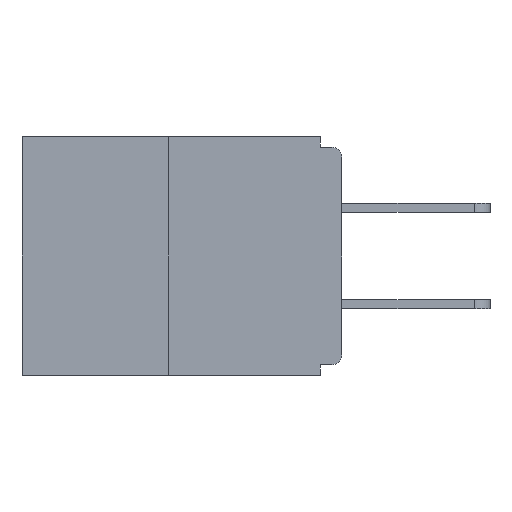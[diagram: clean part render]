
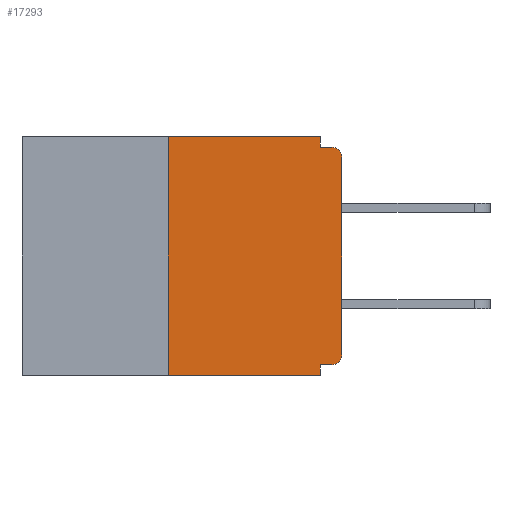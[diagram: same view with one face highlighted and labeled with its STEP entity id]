
A CAD part, left-side view. The second image highlights one B-rep face of the part: STEP entity #17293.
In plain terms, the highlighted planar face has unit normal (-1, 0, 0).
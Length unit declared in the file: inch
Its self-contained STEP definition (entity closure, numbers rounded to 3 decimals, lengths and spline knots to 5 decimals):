
#35 = CARTESIAN_POINT ( 'NONE',  ( 0., 0.25, 0. ) ) ;
#37 = ORIENTED_EDGE ( 'NONE', *, *, #15810, .F. ) ;
#222 = LINE ( 'NONE', #5067, #6453 ) ;
#289 = VECTOR ( 'NONE', #467, 39.37008 ) ;
#467 = DIRECTION ( 'NONE',  ( 0., 1., 0. ) ) ;
#476 = CARTESIAN_POINT ( 'NONE',  ( 0., 0.25, -0.343 ) ) ;
#492 = CARTESIAN_POINT ( 'NONE',  ( 0., 0., -0.015 ) ) ;
#697 = VECTOR ( 'NONE', #11536, 39.37008 ) ;
#717 = VERTEX_POINT ( 'NONE', #6315 ) ;
#784 = AXIS2_PLACEMENT_3D ( 'NONE', #18936, #14417, #8345 ) ;
#836 = LINE ( 'NONE', #3736, #14945 ) ;
#1163 = LINE ( 'NONE', #9948, #697 ) ;
#1172 = CARTESIAN_POINT ( 'NONE',  ( 0., 0., -0.313 ) ) ;
#1773 = EDGE_CURVE ( 'NONE', #6653, #7710, #836, .T. ) ;
#1789 = EDGE_CURVE ( 'NONE', #2468, #10516, #15435, .T. ) ;
#2468 = VERTEX_POINT ( 'NONE', #35 ) ;
#3152 = EDGE_LOOP ( 'NONE', ( #18760, #17387, #11220, #4796, #8653, #9577, #8104, #3454, #37, #15561 ) ) ;
#3274 = DIRECTION ( 'NONE',  ( -1., 0., 0. ) ) ;
#3454 = ORIENTED_EDGE ( 'NONE', *, *, #9477, .T. ) ;
#3498 = CARTESIAN_POINT ( 'NONE',  ( 0., 0., -0.328 ) ) ;
#3604 = DIRECTION ( 'NONE',  ( 0., -1., 0. ) ) ;
#3695 = CARTESIAN_POINT ( 'NONE',  ( 0., 0., 0. ) ) ;
#3736 = CARTESIAN_POINT ( 'NONE',  ( 0., 0.46, -0.343 ) ) ;
#3922 = CARTESIAN_POINT ( 'NONE',  ( 0., 0.46, 0. ) ) ;
#4766 = CARTESIAN_POINT ( 'NONE',  ( 0., 0.015, -0.03 ) ) ;
#4796 = ORIENTED_EDGE ( 'NONE', *, *, #15490, .F. ) ;
#5067 = CARTESIAN_POINT ( 'NONE',  ( 0., 0.031, 0. ) ) ;
#5096 = EDGE_CURVE ( 'NONE', #7377, #13472, #15283, .T. ) ;
#5201 = VECTOR ( 'NONE', #13180, 39.37008 ) ;
#5487 = EDGE_CURVE ( 'NONE', #10516, #18674, #222, .T. ) ;
#5579 = EDGE_CURVE ( 'NONE', #6653, #2468, #1163, .T. ) ;
#6140 = CARTESIAN_POINT ( 'NONE',  ( 0., 0., -0.03 ) ) ;
#6315 = CARTESIAN_POINT ( 'NONE',  ( 0., 0.015, -0.015 ) ) ;
#6453 = VECTOR ( 'NONE', #17282, 39.37008 ) ;
#6653 = VERTEX_POINT ( 'NONE', #476 ) ;
#6843 = AXIS2_PLACEMENT_3D ( 'NONE', #8447, #19269, #14647 ) ;
#7377 = VERTEX_POINT ( 'NONE', #18433 ) ;
#7611 = AXIS2_PLACEMENT_3D ( 'NONE', #4766, #3274, #15344 ) ;
#7710 = VERTEX_POINT ( 'NONE', #18407 ) ;
#8104 = ORIENTED_EDGE ( 'NONE', *, *, #18426, .T. ) ;
#8345 = DIRECTION ( 'NONE',  ( 0., 0., -1. ) ) ;
#8407 = DIRECTION ( 'NONE',  ( 0., 0., 1. ) ) ;
#8447 = CARTESIAN_POINT ( 'NONE',  ( 0., 0.46, 0. ) ) ;
#8653 = ORIENTED_EDGE ( 'NONE', *, *, #18342, .F. ) ;
#9157 = VECTOR ( 'NONE', #8407, 39.37008 ) ;
#9477 = EDGE_CURVE ( 'NONE', #18735, #717, #11991, .T. ) ;
#9518 = VECTOR ( 'NONE', #10223, 39.37008 ) ;
#9577 = ORIENTED_EDGE ( 'NONE', *, *, #5096, .T. ) ;
#9948 = CARTESIAN_POINT ( 'NONE',  ( 0., 0.25, 0. ) ) ;
#10217 = LINE ( 'NONE', #492, #19510 ) ;
#10223 = DIRECTION ( 'NONE',  ( 0., 0., -1. ) ) ;
#10516 = VERTEX_POINT ( 'NONE', #17755 ) ;
#11220 = ORIENTED_EDGE ( 'NONE', *, *, #1773, .T. ) ;
#11402 = DIRECTION ( 'NONE',  ( 0., -1., 0. ) ) ;
#11536 = DIRECTION ( 'NONE',  ( 0., 0., 1. ) ) ;
#11818 = VERTEX_POINT ( 'NONE', #12391 ) ;
#11991 = CIRCLE ( 'NONE', #7611, 0.015 ) ;
#12029 = LINE ( 'NONE', #3498, #289 ) ;
#12391 = CARTESIAN_POINT ( 'NONE',  ( 0., 0.031, -0.328 ) ) ;
#12835 = LINE ( 'NONE', #18020, #9518 ) ;
#13180 = DIRECTION ( 'NONE',  ( 0., -1., 0. ) ) ;
#13472 = VERTEX_POINT ( 'NONE', #1172 ) ;
#14417 = DIRECTION ( 'NONE',  ( -1., 0., 0. ) ) ;
#14647 = DIRECTION ( 'NONE',  ( 0., 0., -1. ) ) ;
#14945 = VECTOR ( 'NONE', #3604, 39.37008 ) ;
#15283 = CIRCLE ( 'NONE', #784, 0.015 ) ;
#15344 = DIRECTION ( 'NONE',  ( 0., 0., -1. ) ) ;
#15435 = LINE ( 'NONE', #3922, #5201 ) ;
#15490 = EDGE_CURVE ( 'NONE', #11818, #7710, #12835, .T. ) ;
#15561 = ORIENTED_EDGE ( 'NONE', *, *, #5487, .F. ) ;
#15810 = EDGE_CURVE ( 'NONE', #18674, #717, #10217, .T. ) ;
#16589 = FACE_OUTER_BOUND ( 'NONE', #3152, .T. ) ;
#17282 = DIRECTION ( 'NONE',  ( 0., 0., -1. ) ) ;
#17293 = ADVANCED_FACE ( 'NONE', ( #16589 ), #17549, .F. ) ;
#17387 = ORIENTED_EDGE ( 'NONE', *, *, #5579, .F. ) ;
#17549 = PLANE ( 'NONE',  #6843 ) ;
#17755 = CARTESIAN_POINT ( 'NONE',  ( 0., 0.031, 0. ) ) ;
#18020 = CARTESIAN_POINT ( 'NONE',  ( 0., 0.031, -0.343 ) ) ;
#18240 = LINE ( 'NONE', #3695, #9157 ) ;
#18306 = CARTESIAN_POINT ( 'NONE',  ( 0., 0.031, -0.015 ) ) ;
#18342 = EDGE_CURVE ( 'NONE', #7377, #11818, #12029, .T. ) ;
#18407 = CARTESIAN_POINT ( 'NONE',  ( 0., 0.031, -0.343 ) ) ;
#18426 = EDGE_CURVE ( 'NONE', #13472, #18735, #18240, .T. ) ;
#18433 = CARTESIAN_POINT ( 'NONE',  ( 0., 0.015, -0.328 ) ) ;
#18674 = VERTEX_POINT ( 'NONE', #18306 ) ;
#18735 = VERTEX_POINT ( 'NONE', #6140 ) ;
#18760 = ORIENTED_EDGE ( 'NONE', *, *, #1789, .F. ) ;
#18936 = CARTESIAN_POINT ( 'NONE',  ( 0., 0.015, -0.313 ) ) ;
#19269 = DIRECTION ( 'NONE',  ( 1., 0., 0. ) ) ;
#19510 = VECTOR ( 'NONE', #11402, 39.37008 ) ;
